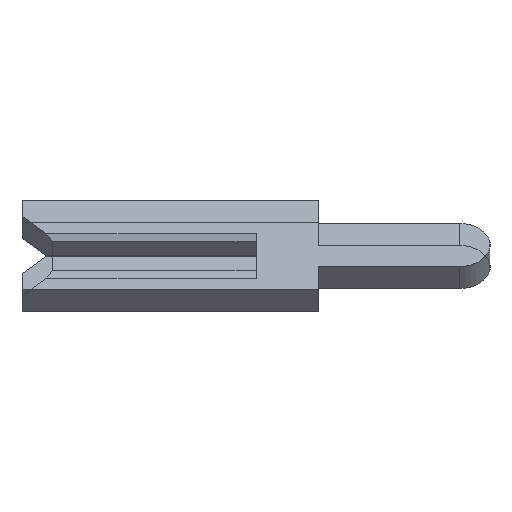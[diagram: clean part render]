
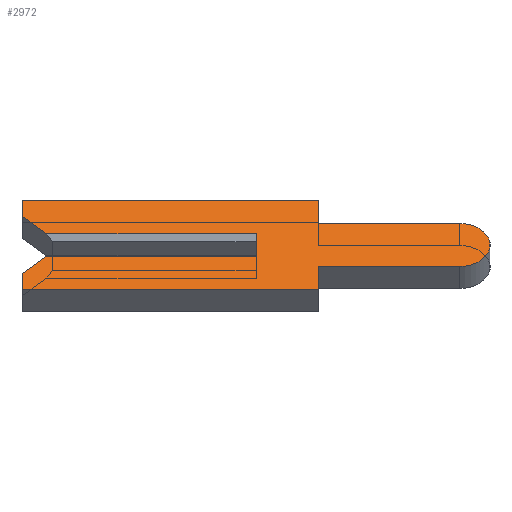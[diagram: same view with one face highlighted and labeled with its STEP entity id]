
A CAD part, left-side view. The second image highlights one B-rep face of the part: STEP entity #2972.
In plain terms, the highlighted face is planar.
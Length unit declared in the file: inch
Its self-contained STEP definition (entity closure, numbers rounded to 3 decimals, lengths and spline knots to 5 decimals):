
#84 = CARTESIAN_POINT ( 'NONE',  ( -0.01, -0.04, 0.04 ) ) ;
#141 = VERTEX_POINT ( 'NONE', #3442 ) ;
#145 = DIRECTION ( 'NONE',  ( 0., -0.707, 0.707 ) ) ;
#172 = CARTESIAN_POINT ( 'NONE',  ( -0.01, 0.15, -0.04 ) ) ;
#179 = LINE ( 'NONE', #1600, #2090 ) ;
#207 = DIRECTION ( 'NONE',  ( 0., -1., 0. ) ) ;
#227 = DIRECTION ( 'NONE',  ( 0., 0.707, 0.707 ) ) ;
#233 = AXIS2_PLACEMENT_3D ( 'NONE', #2521, #1638, #2834 ) ;
#240 = VECTOR ( 'NONE', #3742, 39.37008 ) ;
#260 = CARTESIAN_POINT ( 'NONE',  ( -0.01, -0.04, 0.0195 ) ) ;
#269 = LINE ( 'NONE', #2641, #3786 ) ;
#287 = ORIENTED_EDGE ( 'NONE', *, *, #3750, .F. ) ;
#357 = LINE ( 'NONE', #2148, #2701 ) ;
#361 = VERTEX_POINT ( 'NONE', #734 ) ;
#371 = ORIENTED_EDGE ( 'NONE', *, *, #3023, .F. ) ;
#404 = CARTESIAN_POINT ( 'NONE',  ( -0.01, -0.1305, 0. ) ) ;
#405 = ORIENTED_EDGE ( 'NONE', *, *, #2869, .F. ) ;
#420 = LINE ( 'NONE', #1986, #3667 ) ;
#442 = LINE ( 'NONE', #1161, #3281 ) ;
#537 = LINE ( 'NONE', #1046, #1202 ) ;
#586 = VERTEX_POINT ( 'NONE', #1684 ) ;
#591 = CIRCLE ( 'NONE', #1163, 0.0195 ) ;
#628 = VECTOR ( 'NONE', #145, 39.37008 ) ;
#669 = CARTESIAN_POINT ( 'NONE',  ( -0.01, -0.04, 0.04 ) ) ;
#713 = CARTESIAN_POINT ( 'NONE',  ( -0.01, 0.15, -0.04 ) ) ;
#724 = EDGE_CURVE ( 'NONE', #1780, #882, #2273, .T. ) ;
#734 = CARTESIAN_POINT ( 'NONE',  ( -0.01, -0.1305, 0.0195 ) ) ;
#784 = DIRECTION ( 'NONE',  ( 0., -1., 0. ) ) ;
#785 = ORIENTED_EDGE ( 'NONE', *, *, #3256, .T. ) ;
#827 = CARTESIAN_POINT ( 'NONE',  ( -0.01, 0.15, 0.04 ) ) ;
#882 = VERTEX_POINT ( 'NONE', #827 ) ;
#913 = LINE ( 'NONE', #2548, #628 ) ;
#918 = ORIENTED_EDGE ( 'NONE', *, *, #3803, .F. ) ;
#952 = DIRECTION ( 'NONE',  ( 1., 0., 0. ) ) ;
#972 = EDGE_CURVE ( 'NONE', #2773, #3420, #357, .T. ) ;
#1034 = ORIENTED_EDGE ( 'NONE', *, *, #1730, .F. ) ;
#1046 = CARTESIAN_POINT ( 'NONE',  ( -0.01, 0.15, 0.01 ) ) ;
#1063 = LINE ( 'NONE', #84, #2186 ) ;
#1118 = LINE ( 'NONE', #3431, #2130 ) ;
#1161 = CARTESIAN_POINT ( 'NONE',  ( -0.01, -0.04, -0.0195 ) ) ;
#1163 = AXIS2_PLACEMENT_3D ( 'NONE', #404, #952, #3056 ) ;
#1202 = VECTOR ( 'NONE', #3751, 39.37008 ) ;
#1208 = ORIENTED_EDGE ( 'NONE', *, *, #3280, .F. ) ;
#1251 = LINE ( 'NONE', #2463, #1945 ) ;
#1257 = EDGE_CURVE ( 'NONE', #1719, #361, #269, .T. ) ;
#1261 = VERTEX_POINT ( 'NONE', #3510 ) ;
#1298 = CARTESIAN_POINT ( 'NONE',  ( -0.01, 0.134, -0.01 ) ) ;
#1372 = CARTESIAN_POINT ( 'NONE',  ( -0.01, -0.04, -0.0195 ) ) ;
#1507 = ORIENTED_EDGE ( 'NONE', *, *, #724, .F. ) ;
#1549 = EDGE_LOOP ( 'NONE', ( #785, #1692, #1590, #1208, #2670, #287, #371, #1034, #2619, #3007, #405, #2457, #1507, #918 ) ) ;
#1590 = ORIENTED_EDGE ( 'NONE', *, *, #972, .F. ) ;
#1600 = CARTESIAN_POINT ( 'NONE',  ( -0.01, 0.15, 0.04 ) ) ;
#1638 = DIRECTION ( 'NONE',  ( 1., 0., 0. ) ) ;
#1679 = DIRECTION ( 'NONE',  ( 0., 0., -1. ) ) ;
#1684 = CARTESIAN_POINT ( 'NONE',  ( -0.01, 0.15, -0.026 ) ) ;
#1692 = ORIENTED_EDGE ( 'NONE', *, *, #2814, .F. ) ;
#1719 = VERTEX_POINT ( 'NONE', #260 ) ;
#1730 = EDGE_CURVE ( 'NONE', #141, #3415, #442, .T. ) ;
#1780 = VERTEX_POINT ( 'NONE', #3567 ) ;
#1831 = LINE ( 'NONE', #172, #240 ) ;
#1945 = VECTOR ( 'NONE', #3378, 39.37008 ) ;
#1982 = DIRECTION ( 'NONE',  ( 0., 0., 1. ) ) ;
#1986 = CARTESIAN_POINT ( 'NONE',  ( -0.01, 0.1305, 0.0065 ) ) ;
#2090 = VECTOR ( 'NONE', #2750, 39.37008 ) ;
#2121 = VECTOR ( 'NONE', #3180, 39.37008 ) ;
#2130 = VECTOR ( 'NONE', #1679, 39.37008 ) ;
#2148 = CARTESIAN_POINT ( 'NONE',  ( -0.01, -0.1305, -0.01 ) ) ;
#2186 = VECTOR ( 'NONE', #3404, 39.37008 ) ;
#2232 = CARTESIAN_POINT ( 'NONE',  ( -0.01, 0., -0.01 ) ) ;
#2273 = LINE ( 'NONE', #3432, #2748 ) ;
#2369 = VERTEX_POINT ( 'NONE', #669 ) ;
#2381 = VERTEX_POINT ( 'NONE', #2478 ) ;
#2457 = ORIENTED_EDGE ( 'NONE', *, *, #2739, .F. ) ;
#2463 = CARTESIAN_POINT ( 'NONE',  ( -0.01, 0., 0.0065 ) ) ;
#2478 = CARTESIAN_POINT ( 'NONE',  ( -0.01, 0., 0.01 ) ) ;
#2521 = CARTESIAN_POINT ( 'NONE',  ( -0.01, -0.1305, 0. ) ) ;
#2548 = CARTESIAN_POINT ( 'NONE',  ( -0.01, 0.1305, -0.0065 ) ) ;
#2619 = ORIENTED_EDGE ( 'NONE', *, *, #2797, .F. ) ;
#2641 = CARTESIAN_POINT ( 'NONE',  ( -0.01, -0.04, 0.0195 ) ) ;
#2670 = ORIENTED_EDGE ( 'NONE', *, *, #3146, .F. ) ;
#2701 = VECTOR ( 'NONE', #207, 39.37008 ) ;
#2739 = EDGE_CURVE ( 'NONE', #882, #2369, #179, .T. ) ;
#2748 = VECTOR ( 'NONE', #1982, 39.37008 ) ;
#2750 = DIRECTION ( 'NONE',  ( 0., -1., 0. ) ) ;
#2773 = VERTEX_POINT ( 'NONE', #1298 ) ;
#2797 = EDGE_CURVE ( 'NONE', #361, #141, #591, .T. ) ;
#2814 = EDGE_CURVE ( 'NONE', #3420, #2381, #1251, .T. ) ;
#2834 = DIRECTION ( 'NONE',  ( 0., 0., -1. ) ) ;
#2869 = EDGE_CURVE ( 'NONE', #2369, #1719, #1063, .T. ) ;
#2913 = VERTEX_POINT ( 'NONE', #3776 ) ;
#2972 = ADVANCED_FACE ( 'NONE', ( #3081 ), #3470, .F. ) ;
#3007 = ORIENTED_EDGE ( 'NONE', *, *, #1257, .F. ) ;
#3023 = EDGE_CURVE ( 'NONE', #3415, #2913, #1118, .T. ) ;
#3047 = VERTEX_POINT ( 'NONE', #713 ) ;
#3056 = DIRECTION ( 'NONE',  ( 0., 0., -1. ) ) ;
#3081 = FACE_OUTER_BOUND ( 'NONE', #1549, .T. ) ;
#3146 = EDGE_CURVE ( 'NONE', #3047, #586, #3738, .T. ) ;
#3180 = DIRECTION ( 'NONE',  ( 0., 0., 1. ) ) ;
#3256 = EDGE_CURVE ( 'NONE', #1261, #2381, #537, .T. ) ;
#3270 = DIRECTION ( 'NONE',  ( 0., 1., 0. ) ) ;
#3280 = EDGE_CURVE ( 'NONE', #586, #2773, #913, .T. ) ;
#3281 = VECTOR ( 'NONE', #3270, 39.37008 ) ;
#3378 = DIRECTION ( 'NONE',  ( 0., 0., 1. ) ) ;
#3404 = DIRECTION ( 'NONE',  ( 0., 0., -1. ) ) ;
#3415 = VERTEX_POINT ( 'NONE', #1372 ) ;
#3420 = VERTEX_POINT ( 'NONE', #2232 ) ;
#3431 = CARTESIAN_POINT ( 'NONE',  ( -0.01, -0.04, -0.04 ) ) ;
#3432 = CARTESIAN_POINT ( 'NONE',  ( -0.01, 0.15, 0.026 ) ) ;
#3442 = CARTESIAN_POINT ( 'NONE',  ( -0.01, -0.1305, -0.0195 ) ) ;
#3447 = CARTESIAN_POINT ( 'NONE',  ( -0.01, 0.15, -0.026 ) ) ;
#3470 = PLANE ( 'NONE',  #233 ) ;
#3510 = CARTESIAN_POINT ( 'NONE',  ( -0.01, 0.134, 0.01 ) ) ;
#3567 = CARTESIAN_POINT ( 'NONE',  ( -0.01, 0.15, 0.026 ) ) ;
#3667 = VECTOR ( 'NONE', #227, 39.37008 ) ;
#3738 = LINE ( 'NONE', #3447, #2121 ) ;
#3742 = DIRECTION ( 'NONE',  ( 0., 1., 0. ) ) ;
#3750 = EDGE_CURVE ( 'NONE', #2913, #3047, #1831, .T. ) ;
#3751 = DIRECTION ( 'NONE',  ( 0., -1., 0. ) ) ;
#3776 = CARTESIAN_POINT ( 'NONE',  ( -0.01, -0.04, -0.04 ) ) ;
#3786 = VECTOR ( 'NONE', #784, 39.37008 ) ;
#3803 = EDGE_CURVE ( 'NONE', #1261, #1780, #420, .T. ) ;
